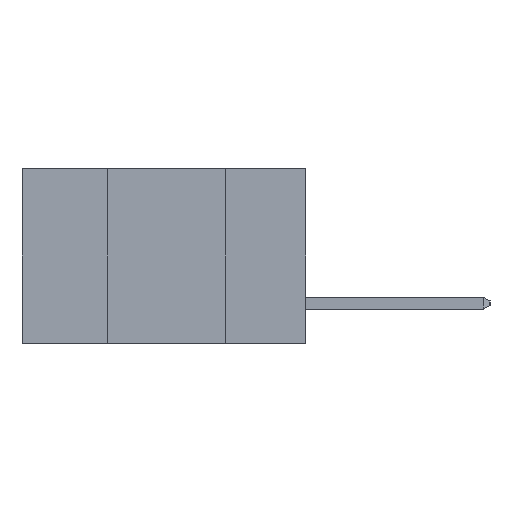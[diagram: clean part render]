
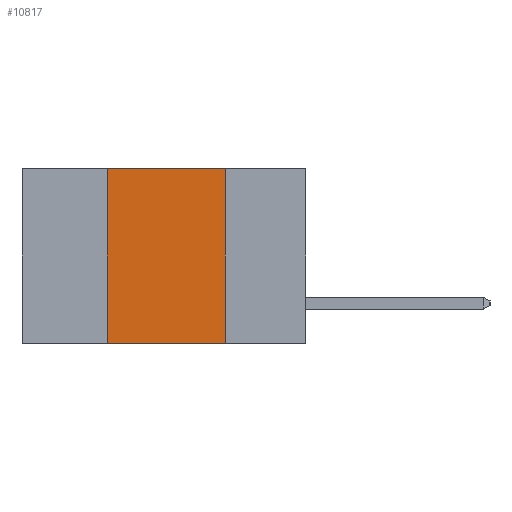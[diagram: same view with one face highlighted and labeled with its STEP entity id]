
A CAD part, left-side view. The second image highlights one B-rep face of the part: STEP entity #10817.
In plain terms, the highlighted planar face has unit normal (-1, 0, 0).
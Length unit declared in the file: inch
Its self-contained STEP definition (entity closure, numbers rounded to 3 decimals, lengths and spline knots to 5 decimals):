
#84 = EDGE_CURVE ( 'NONE', #4538, #15082, #15175, .T. ) ;
#218 = ORIENTED_EDGE ( 'NONE', *, *, #84, .F. ) ;
#846 = DIRECTION ( 'NONE',  ( 0., 0., 1. ) ) ;
#943 = ORIENTED_EDGE ( 'NONE', *, *, #13678, .T. ) ;
#1027 = VERTEX_POINT ( 'NONE', #12692 ) ;
#1435 = LINE ( 'NONE', #3268, #14739 ) ;
#1660 = DIRECTION ( 'NONE',  ( 0., -1., 0. ) ) ;
#1850 = ORIENTED_EDGE ( 'NONE', *, *, #7702, .F. ) ;
#2342 = VECTOR ( 'NONE', #1660, 39.37008 ) ;
#2443 = CARTESIAN_POINT ( 'NONE',  ( 0., 0.42, 0. ) ) ;
#2623 = CARTESIAN_POINT ( 'NONE',  ( 0., 0.6, 0. ) ) ;
#2962 = VERTEX_POINT ( 'NONE', #4331 ) ;
#3041 = ORIENTED_EDGE ( 'NONE', *, *, #10266, .F. ) ;
#3268 = CARTESIAN_POINT ( 'NONE',  ( 0., 0.17, 0. ) ) ;
#3350 = CARTESIAN_POINT ( 'NONE',  ( 0., 0.6, 0. ) ) ;
#4268 = LINE ( 'NONE', #7475, #13699 ) ;
#4331 = CARTESIAN_POINT ( 'NONE',  ( 0., 0.42, -0.37 ) ) ;
#4538 = VERTEX_POINT ( 'NONE', #2443 ) ;
#5116 = FACE_OUTER_BOUND ( 'NONE', #8559, .T. ) ;
#6036 = PLANE ( 'NONE',  #14731 ) ;
#6746 = VECTOR ( 'NONE', #12228, 39.37008 ) ;
#7150 = LINE ( 'NONE', #14661, #6746 ) ;
#7336 = DIRECTION ( 'NONE',  ( 0., 0., -1. ) ) ;
#7475 = CARTESIAN_POINT ( 'NONE',  ( 0., 0.42, 0. ) ) ;
#7702 = EDGE_CURVE ( 'NONE', #15082, #1027, #1435, .T. ) ;
#8559 = EDGE_LOOP ( 'NONE', ( #1850, #218, #3041, #943 ) ) ;
#10266 = EDGE_CURVE ( 'NONE', #2962, #4538, #4268, .T. ) ;
#10817 = ADVANCED_FACE ( 'NONE', ( #5116 ), #6036, .F. ) ;
#12228 = DIRECTION ( 'NONE',  ( 0., -1., 0. ) ) ;
#12692 = CARTESIAN_POINT ( 'NONE',  ( 0., 0.17, -0.37 ) ) ;
#13587 = DIRECTION ( 'NONE',  ( 0., 0., -1. ) ) ;
#13678 = EDGE_CURVE ( 'NONE', #2962, #1027, #7150, .T. ) ;
#13699 = VECTOR ( 'NONE', #846, 39.37008 ) ;
#14531 = CARTESIAN_POINT ( 'NONE',  ( 0., 0.17, 0. ) ) ;
#14661 = CARTESIAN_POINT ( 'NONE',  ( 0., 0.6, -0.37 ) ) ;
#14731 = AXIS2_PLACEMENT_3D ( 'NONE', #3350, #14855, #7336 ) ;
#14739 = VECTOR ( 'NONE', #13587, 39.37008 ) ;
#14855 = DIRECTION ( 'NONE',  ( 1., 0., 0. ) ) ;
#15082 = VERTEX_POINT ( 'NONE', #14531 ) ;
#15175 = LINE ( 'NONE', #2623, #2342 ) ;
